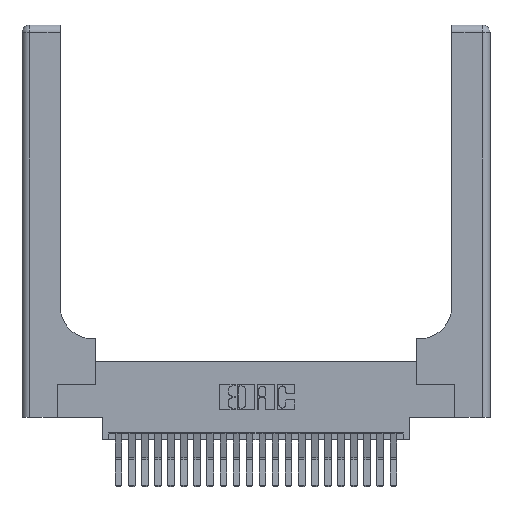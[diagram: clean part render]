
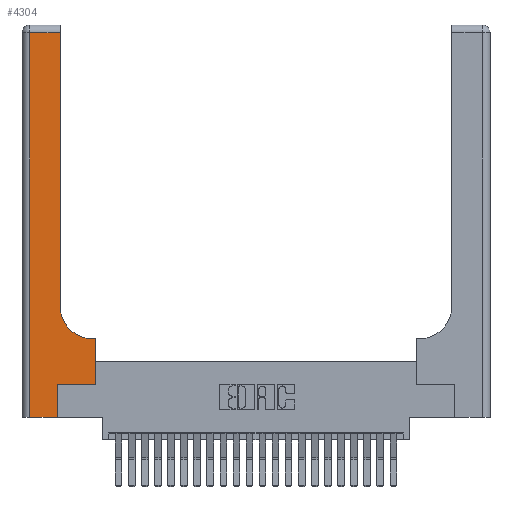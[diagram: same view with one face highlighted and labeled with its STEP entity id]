
A CAD part, top view. The second image highlights one B-rep face of the part: STEP entity #4304.
In plain terms, the highlighted planar face has unit normal (0, 0, 1).
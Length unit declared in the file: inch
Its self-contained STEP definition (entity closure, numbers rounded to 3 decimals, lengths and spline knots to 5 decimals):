
#103 = EDGE_LOOP ( 'NONE', ( #20049, #10742, #239, #11067, #20344, #7653, #1607, #18065, #861 ) ) ;
#214 = DIRECTION ( 'NONE',  ( 1., 0., 0. ) ) ;
#239 = ORIENTED_EDGE ( 'NONE', *, *, #16414, .T. ) ;
#851 = VECTOR ( 'NONE', #24900, 39.37008 ) ;
#861 = ORIENTED_EDGE ( 'NONE', *, *, #21993, .T. ) ;
#931 = DIRECTION ( 'NONE',  ( 0., 1., 0. ) ) ;
#1136 = CARTESIAN_POINT ( 'NONE',  ( 0.269, 0., 0.37 ) ) ;
#1163 = CIRCLE ( 'NONE', #24885, 0.25 ) ;
#1238 = CARTESIAN_POINT ( 'NONE',  ( 0., 3., 0.37 ) ) ;
#1607 = ORIENTED_EDGE ( 'NONE', *, *, #7137, .T. ) ;
#2544 = VERTEX_POINT ( 'NONE', #18014 ) ;
#2726 = CARTESIAN_POINT ( 'NONE',  ( 0.5415, 0.85, 0.37 ) ) ;
#3168 = VECTOR ( 'NONE', #931, 39.37008 ) ;
#3712 = CARTESIAN_POINT ( 'NONE',  ( 0.2915, 0.85, 0.37 ) ) ;
#4163 = VECTOR ( 'NONE', #5381, 39.37008 ) ;
#4304 = ADVANCED_FACE ( 'NONE', ( #10245 ), #20923, .F. ) ;
#4446 = LINE ( 'NONE', #16651, #14888 ) ;
#4685 = VERTEX_POINT ( 'NONE', #16534 ) ;
#5381 = DIRECTION ( 'NONE',  ( 0., 1., 0. ) ) ;
#6382 = CARTESIAN_POINT ( 'NONE',  ( 0.269, 0.25, 0.37 ) ) ;
#6582 = VECTOR ( 'NONE', #22906, 39.37008 ) ;
#7137 = EDGE_CURVE ( 'NONE', #20030, #13897, #22689, .T. ) ;
#7653 = ORIENTED_EDGE ( 'NONE', *, *, #11582, .T. ) ;
#7756 = VERTEX_POINT ( 'NONE', #1136 ) ;
#7968 = VERTEX_POINT ( 'NONE', #3712 ) ;
#8354 = EDGE_CURVE ( 'NONE', #14729, #7756, #11870, .T. ) ;
#8449 = EDGE_CURVE ( 'NONE', #13897, #24001, #9437, .T. ) ;
#9169 = DIRECTION ( 'NONE',  ( 0., 0., -1. ) ) ;
#9437 = LINE ( 'NONE', #13511, #10644 ) ;
#10013 = CARTESIAN_POINT ( 'NONE',  ( 0.06, 0., 0.37 ) ) ;
#10221 = DIRECTION ( 'NONE',  ( 1., 0., 0. ) ) ;
#10245 = FACE_OUTER_BOUND ( 'NONE', #103, .T. ) ;
#10405 = CARTESIAN_POINT ( 'NONE',  ( 0.5585, 0.25, 0.37 ) ) ;
#10644 = VECTOR ( 'NONE', #17108, 39.37008 ) ;
#10742 = ORIENTED_EDGE ( 'NONE', *, *, #16494, .T. ) ;
#11067 = ORIENTED_EDGE ( 'NONE', *, *, #8354, .T. ) ;
#11582 = EDGE_CURVE ( 'NONE', #4685, #20030, #15749, .T. ) ;
#11870 = LINE ( 'NONE', #18807, #851 ) ;
#12078 = DIRECTION ( 'NONE',  ( 0., 1., 0. ) ) ;
#12566 = CARTESIAN_POINT ( 'NONE',  ( 0.2915, 3., 0.37 ) ) ;
#13148 = CARTESIAN_POINT ( 'NONE',  ( 0.5415, 0.6, 0.37 ) ) ;
#13511 = CARTESIAN_POINT ( 'NONE',  ( 0.2915, 0.6, 0.37 ) ) ;
#13897 = VERTEX_POINT ( 'NONE', #14895 ) ;
#14575 = LINE ( 'NONE', #15057, #4163 ) ;
#14729 = VERTEX_POINT ( 'NONE', #10013 ) ;
#14888 = VECTOR ( 'NONE', #18447, 39.37008 ) ;
#14895 = CARTESIAN_POINT ( 'NONE',  ( 0.5585, 0.6, 0.37 ) ) ;
#15057 = CARTESIAN_POINT ( 'NONE',  ( 0.269, 0., 0.37 ) ) ;
#15749 = LINE ( 'NONE', #6382, #18483 ) ;
#15821 = EDGE_CURVE ( 'NONE', #7756, #4685, #14575, .T. ) ;
#16414 = EDGE_CURVE ( 'NONE', #22053, #14729, #4446, .T. ) ;
#16419 = LINE ( 'NONE', #23082, #6582 ) ;
#16494 = EDGE_CURVE ( 'NONE', #2544, #22053, #16419, .T. ) ;
#16534 = CARTESIAN_POINT ( 'NONE',  ( 0.269, 0.25, 0.37 ) ) ;
#16651 = CARTESIAN_POINT ( 'NONE',  ( 0.06, 3., 0.37 ) ) ;
#17108 = DIRECTION ( 'NONE',  ( -1., 0., 0. ) ) ;
#18014 = CARTESIAN_POINT ( 'NONE',  ( 0.2915, 2.94, 0.37 ) ) ;
#18065 = ORIENTED_EDGE ( 'NONE', *, *, #8449, .T. ) ;
#18113 = DIRECTION ( 'NONE',  ( 0., 0., -1. ) ) ;
#18447 = DIRECTION ( 'NONE',  ( 0., -1., 0. ) ) ;
#18483 = VECTOR ( 'NONE', #214, 39.37008 ) ;
#18807 = CARTESIAN_POINT ( 'NONE',  ( 0., 0., 0.37 ) ) ;
#20030 = VERTEX_POINT ( 'NONE', #10405 ) ;
#20049 = ORIENTED_EDGE ( 'NONE', *, *, #24455, .T. ) ;
#20344 = ORIENTED_EDGE ( 'NONE', *, *, #15821, .T. ) ;
#20758 = AXIS2_PLACEMENT_3D ( 'NONE', #1238, #9169, #22905 ) ;
#20923 = PLANE ( 'NONE',  #20758 ) ;
#21167 = VECTOR ( 'NONE', #12078, 39.37008 ) ;
#21993 = EDGE_CURVE ( 'NONE', #24001, #7968, #1163, .T. ) ;
#22053 = VERTEX_POINT ( 'NONE', #23858 ) ;
#22689 = LINE ( 'NONE', #23841, #21167 ) ;
#22905 = DIRECTION ( 'NONE',  ( -1., 0., 0. ) ) ;
#22906 = DIRECTION ( 'NONE',  ( -1., 0., 0. ) ) ;
#23082 = CARTESIAN_POINT ( 'NONE',  ( 0., 2.94, 0.37 ) ) ;
#23841 = CARTESIAN_POINT ( 'NONE',  ( 0.5585, 0.25, 0.37 ) ) ;
#23858 = CARTESIAN_POINT ( 'NONE',  ( 0.06, 2.94, 0.37 ) ) ;
#24001 = VERTEX_POINT ( 'NONE', #13148 ) ;
#24455 = EDGE_CURVE ( 'NONE', #7968, #2544, #24926, .T. ) ;
#24885 = AXIS2_PLACEMENT_3D ( 'NONE', #2726, #18113, #10221 ) ;
#24900 = DIRECTION ( 'NONE',  ( 1., 0., 0. ) ) ;
#24926 = LINE ( 'NONE', #12566, #3168 ) ;
